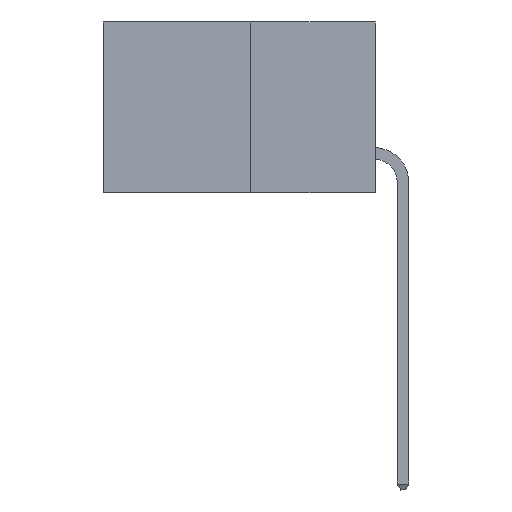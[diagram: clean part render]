
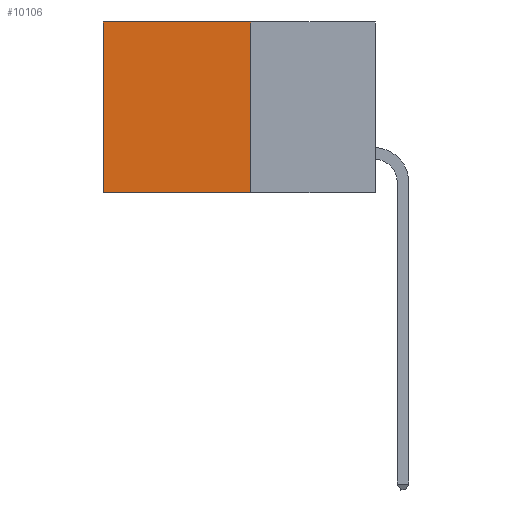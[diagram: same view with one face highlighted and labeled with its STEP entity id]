
A CAD part, left-side view. The second image highlights one B-rep face of the part: STEP entity #10106.
In plain terms, the highlighted planar face has unit normal (-1, 0, 0).
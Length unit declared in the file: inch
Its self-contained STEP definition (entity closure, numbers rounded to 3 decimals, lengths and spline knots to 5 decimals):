
#8 = VECTOR ( 'NONE', #7921, 39.37008 ) ;
#169 = AXIS2_PLACEMENT_3D ( 'NONE', #15183, #769, #9434 ) ;
#581 = CARTESIAN_POINT ( 'NONE',  ( 0.277, 0.59, -0.37 ) ) ;
#769 = DIRECTION ( 'NONE',  ( 1., 0., 0. ) ) ;
#792 = DIRECTION ( 'NONE',  ( 0., 0., -1. ) ) ;
#1689 = FACE_OUTER_BOUND ( 'NONE', #14531, .T. ) ;
#1696 = CARTESIAN_POINT ( 'NONE',  ( 0.277, 0.59, -0.37 ) ) ;
#2639 = ORIENTED_EDGE ( 'NONE', *, *, #9951, .T. ) ;
#2847 = ORIENTED_EDGE ( 'NONE', *, *, #13975, .F. ) ;
#2892 = CARTESIAN_POINT ( 'NONE',  ( 0.277, 0.27, -0.37 ) ) ;
#3006 = LINE ( 'NONE', #9115, #3815 ) ;
#3266 = CARTESIAN_POINT ( 'NONE',  ( 0.277, 0.59, 0. ) ) ;
#3815 = VECTOR ( 'NONE', #10327, 39.37008 ) ;
#4031 = ORIENTED_EDGE ( 'NONE', *, *, #7005, .F. ) ;
#4047 = LINE ( 'NONE', #1696, #10580 ) ;
#4303 = ORIENTED_EDGE ( 'NONE', *, *, #13220, .T. ) ;
#5776 = CARTESIAN_POINT ( 'NONE',  ( 0.277, 0.27, -0.37 ) ) ;
#6271 = LINE ( 'NONE', #14869, #8 ) ;
#6713 = VECTOR ( 'NONE', #792, 39.37008 ) ;
#6997 = PLANE ( 'NONE',  #169 ) ;
#7005 = EDGE_CURVE ( 'NONE', #10290, #11529, #6271, .T. ) ;
#7110 = LINE ( 'NONE', #5776, #6713 ) ;
#7296 = VERTEX_POINT ( 'NONE', #3266 ) ;
#7921 = DIRECTION ( 'NONE',  ( 0., 1., 0. ) ) ;
#8703 = CARTESIAN_POINT ( 'NONE',  ( 0.277, 0.27, 0. ) ) ;
#9115 = CARTESIAN_POINT ( 'NONE',  ( 0.277, 0.27, 0. ) ) ;
#9434 = DIRECTION ( 'NONE',  ( 0., 0., -1. ) ) ;
#9951 = EDGE_CURVE ( 'NONE', #7296, #11529, #4047, .T. ) ;
#10106 = ADVANCED_FACE ( 'NONE', ( #1689 ), #6997, .F. ) ;
#10290 = VERTEX_POINT ( 'NONE', #2892 ) ;
#10327 = DIRECTION ( 'NONE',  ( 0., 1., 0. ) ) ;
#10580 = VECTOR ( 'NONE', #13734, 39.37008 ) ;
#11529 = VERTEX_POINT ( 'NONE', #581 ) ;
#13220 = EDGE_CURVE ( 'NONE', #14418, #7296, #3006, .T. ) ;
#13734 = DIRECTION ( 'NONE',  ( 0., 0., -1. ) ) ;
#13975 = EDGE_CURVE ( 'NONE', #14418, #10290, #7110, .T. ) ;
#14418 = VERTEX_POINT ( 'NONE', #8703 ) ;
#14531 = EDGE_LOOP ( 'NONE', ( #2639, #4031, #2847, #4303 ) ) ;
#14869 = CARTESIAN_POINT ( 'NONE',  ( 0.277, 0.27, -0.37 ) ) ;
#15183 = CARTESIAN_POINT ( 'NONE',  ( 0.277, 0.27, -0.37 ) ) ;
